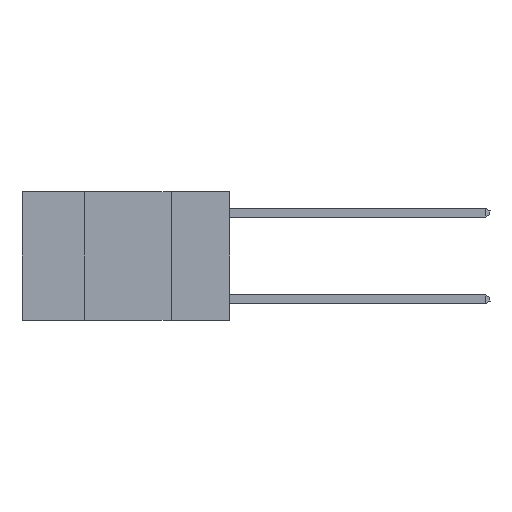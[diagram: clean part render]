
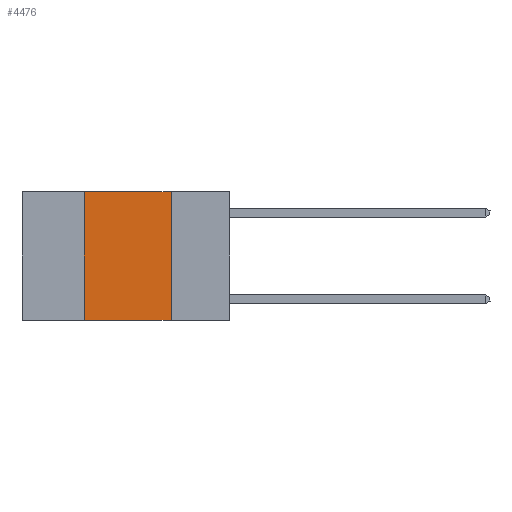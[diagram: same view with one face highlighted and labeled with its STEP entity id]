
A CAD part, left-side view. The second image highlights one B-rep face of the part: STEP entity #4476.
In plain terms, the highlighted planar face has unit normal (-1, 0, 0).
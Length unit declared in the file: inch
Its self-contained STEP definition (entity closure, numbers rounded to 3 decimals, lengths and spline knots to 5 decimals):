
#41 = FACE_OUTER_BOUND ( 'NONE', #15513, .T. ) ;
#79 = VECTOR ( 'NONE', #15031, 39.37008 ) ;
#951 = ORIENTED_EDGE ( 'NONE', *, *, #8718, .F. ) ;
#1167 = VERTEX_POINT ( 'NONE', #17583 ) ;
#1745 = CARTESIAN_POINT ( 'NONE',  ( 0., 0.17, -0.37 ) ) ;
#2155 = DIRECTION ( 'NONE',  ( 0., 0., -1. ) ) ;
#2259 = EDGE_CURVE ( 'NONE', #1167, #13889, #3717, .T. ) ;
#2660 = LINE ( 'NONE', #8182, #16862 ) ;
#3717 = LINE ( 'NONE', #14763, #12298 ) ;
#4476 = ADVANCED_FACE ( 'NONE', ( #41 ), #5565, .F. ) ;
#5132 = ORIENTED_EDGE ( 'NONE', *, *, #9299, .F. ) ;
#5565 = PLANE ( 'NONE',  #10418 ) ;
#7683 = LINE ( 'NONE', #10491, #14689 ) ;
#8182 = CARTESIAN_POINT ( 'NONE',  ( 0., 0.6, 0. ) ) ;
#8191 = CARTESIAN_POINT ( 'NONE',  ( 0., 0.42, 0. ) ) ;
#8203 = CARTESIAN_POINT ( 'NONE',  ( 0., 0.6, 0. ) ) ;
#8378 = DIRECTION ( 'NONE',  ( 1., 0., 0. ) ) ;
#8718 = EDGE_CURVE ( 'NONE', #1167, #15148, #13844, .T. ) ;
#9197 = EDGE_CURVE ( 'NONE', #15148, #13008, #2660, .T. ) ;
#9299 = EDGE_CURVE ( 'NONE', #13008, #13889, #7683, .T. ) ;
#9714 = DIRECTION ( 'NONE',  ( 0., -1., 0. ) ) ;
#10418 = AXIS2_PLACEMENT_3D ( 'NONE', #8203, #8378, #13717 ) ;
#10491 = CARTESIAN_POINT ( 'NONE',  ( 0., 0.17, 0. ) ) ;
#12298 = VECTOR ( 'NONE', #14404, 39.37008 ) ;
#12586 = ORIENTED_EDGE ( 'NONE', *, *, #9197, .F. ) ;
#13008 = VERTEX_POINT ( 'NONE', #17635 ) ;
#13717 = DIRECTION ( 'NONE',  ( 0., 0., -1. ) ) ;
#13844 = LINE ( 'NONE', #16479, #79 ) ;
#13889 = VERTEX_POINT ( 'NONE', #1745 ) ;
#14404 = DIRECTION ( 'NONE',  ( 0., -1., 0. ) ) ;
#14689 = VECTOR ( 'NONE', #2155, 39.37008 ) ;
#14763 = CARTESIAN_POINT ( 'NONE',  ( 0., 0.6, -0.37 ) ) ;
#15031 = DIRECTION ( 'NONE',  ( 0., 0., 1. ) ) ;
#15148 = VERTEX_POINT ( 'NONE', #8191 ) ;
#15336 = ORIENTED_EDGE ( 'NONE', *, *, #2259, .T. ) ;
#15513 = EDGE_LOOP ( 'NONE', ( #5132, #12586, #951, #15336 ) ) ;
#16479 = CARTESIAN_POINT ( 'NONE',  ( 0., 0.42, 0. ) ) ;
#16862 = VECTOR ( 'NONE', #9714, 39.37008 ) ;
#17583 = CARTESIAN_POINT ( 'NONE',  ( 0., 0.42, -0.37 ) ) ;
#17635 = CARTESIAN_POINT ( 'NONE',  ( 0., 0.17, 0. ) ) ;
